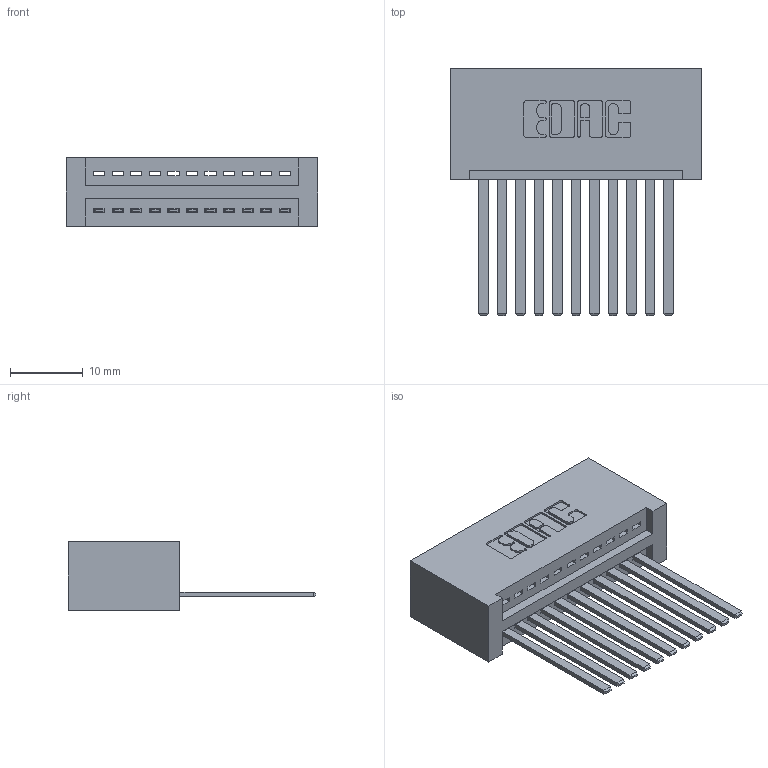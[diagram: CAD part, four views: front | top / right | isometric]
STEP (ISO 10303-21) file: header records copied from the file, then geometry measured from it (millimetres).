
FILE_DESCRIPTION (( 'STEP AP203' ), '1' );
FILE_NAME ('395-011-544-101.STEP', '2018-11-05T15:54:47', ( '' ), ( '' ), 'SwSTEP 2.0', 'SolidWorks 2016', '' );
FILE_SCHEMA (( 'CONFIG_CONTROL_DESIGN' ));
Length unit declared in the file: inch
Products named in the file (3): 345-292-001_345-293-144; 395-011-544-101; 345 Part_No Mounting Lugs
Assembly tree (12 placements, depth 2):
  395-011-544-101
    345 Part_No Mounting Lugs
    345-292-001_345-293-144  x11
Bounding box: 34.54 x 33.96 x 9.4 mm (x, y, z)
Volume: 3738.8 mm3; surface area: 5119.8 mm2
Topology: 12 solids, 12 shells, 690 faces, 2055 edges, 1354 vertices
Faces by surface type: plane 472, cylinder 218
Entity records: 11991 total; most frequent: CARTESIAN_POINT 2085, ORIENTED_EDGE 2030, DIRECTION 1857, EDGE_CURVE 1015, LINE 851, VECTOR 851, VERTEX_POINT 674, AXIS2_PLACEMENT_3D 503
